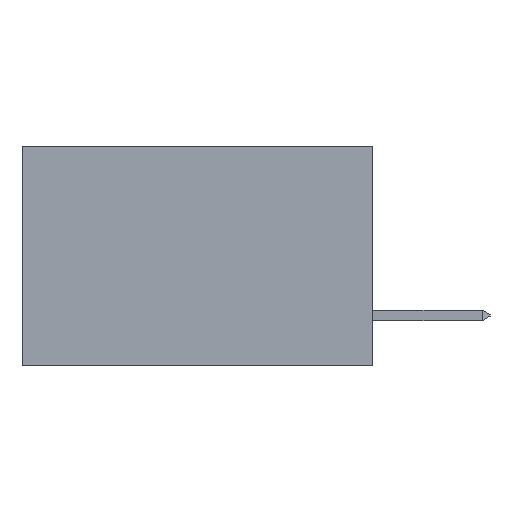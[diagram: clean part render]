
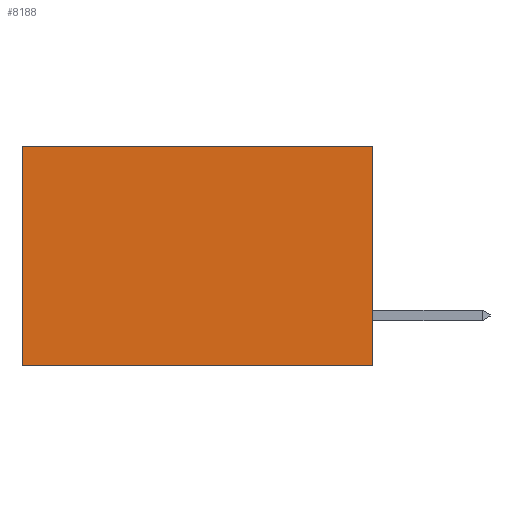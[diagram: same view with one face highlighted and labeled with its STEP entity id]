
A CAD part, left-side view. The second image highlights one B-rep face of the part: STEP entity #8188.
In plain terms, the highlighted planar face has unit normal (-1, 0, 0).
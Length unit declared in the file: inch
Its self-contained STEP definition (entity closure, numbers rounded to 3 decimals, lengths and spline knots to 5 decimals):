
#688 = DIRECTION ( 'NONE',  ( 0., 1., 0. ) ) ;
#880 = VERTEX_POINT ( 'NONE', #12762 ) ;
#1264 = AXIS2_PLACEMENT_3D ( 'NONE', #15002, #16779, #5640 ) ;
#1626 = CARTESIAN_POINT ( 'NONE',  ( 0.277, 0., 0. ) ) ;
#1767 = PLANE ( 'NONE',  #1264 ) ;
#2452 = EDGE_CURVE ( 'NONE', #3312, #11677, #2550, .T. ) ;
#2550 = LINE ( 'NONE', #13965, #7668 ) ;
#2730 = VECTOR ( 'NONE', #7070, 39.37008 ) ;
#3312 = VERTEX_POINT ( 'NONE', #23829 ) ;
#3990 = VECTOR ( 'NONE', #6130, 39.37008 ) ;
#4587 = LINE ( 'NONE', #5328, #3990 ) ;
#4752 = ORIENTED_EDGE ( 'NONE', *, *, #7179, .T. ) ;
#5061 = EDGE_CURVE ( 'NONE', #7482, #880, #4587, .T. ) ;
#5328 = CARTESIAN_POINT ( 'NONE',  ( 0.277, 0., -0.37 ) ) ;
#5640 = DIRECTION ( 'NONE',  ( 0., 0., -1. ) ) ;
#5817 = LINE ( 'NONE', #8425, #21028 ) ;
#6130 = DIRECTION ( 'NONE',  ( 0., 0., -1. ) ) ;
#6950 = ORIENTED_EDGE ( 'NONE', *, *, #5061, .F. ) ;
#7070 = DIRECTION ( 'NONE',  ( 0., 1., 0. ) ) ;
#7106 = ORIENTED_EDGE ( 'NONE', *, *, #17490, .F. ) ;
#7179 = EDGE_CURVE ( 'NONE', #7482, #3312, #5817, .T. ) ;
#7482 = VERTEX_POINT ( 'NONE', #1626 ) ;
#7668 = VECTOR ( 'NONE', #16219, 39.37008 ) ;
#8166 = ORIENTED_EDGE ( 'NONE', *, *, #2452, .T. ) ;
#8188 = ADVANCED_FACE ( 'NONE', ( #17974 ), #1767, .F. ) ;
#8425 = CARTESIAN_POINT ( 'NONE',  ( 0.277, 0., 0. ) ) ;
#9071 = CARTESIAN_POINT ( 'NONE',  ( 0.277, 0.59, -0.37 ) ) ;
#11677 = VERTEX_POINT ( 'NONE', #9071 ) ;
#12762 = CARTESIAN_POINT ( 'NONE',  ( 0.277, 0., -0.37 ) ) ;
#13965 = CARTESIAN_POINT ( 'NONE',  ( 0.277, 0.59, -0.37 ) ) ;
#15002 = CARTESIAN_POINT ( 'NONE',  ( 0.277, 0., -0.37 ) ) ;
#16219 = DIRECTION ( 'NONE',  ( 0., 0., -1. ) ) ;
#16779 = DIRECTION ( 'NONE',  ( 1., 0., 0. ) ) ;
#17490 = EDGE_CURVE ( 'NONE', #880, #11677, #21767, .T. ) ;
#17974 = FACE_OUTER_BOUND ( 'NONE', #23259, .T. ) ;
#19889 = CARTESIAN_POINT ( 'NONE',  ( 0.277, 0., -0.37 ) ) ;
#21028 = VECTOR ( 'NONE', #688, 39.37008 ) ;
#21767 = LINE ( 'NONE', #19889, #2730 ) ;
#23259 = EDGE_LOOP ( 'NONE', ( #8166, #7106, #6950, #4752 ) ) ;
#23829 = CARTESIAN_POINT ( 'NONE',  ( 0.277, 0.59, 0. ) ) ;
